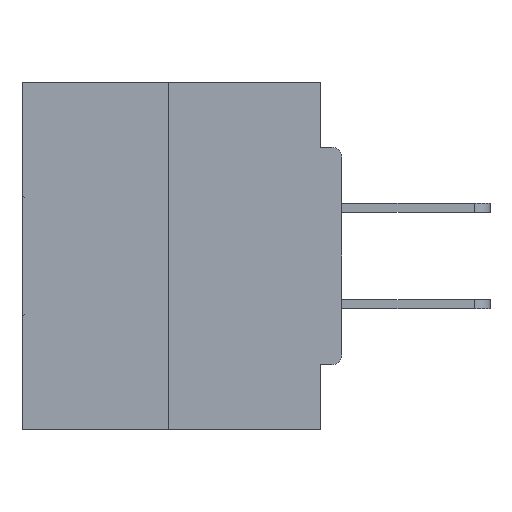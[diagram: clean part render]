
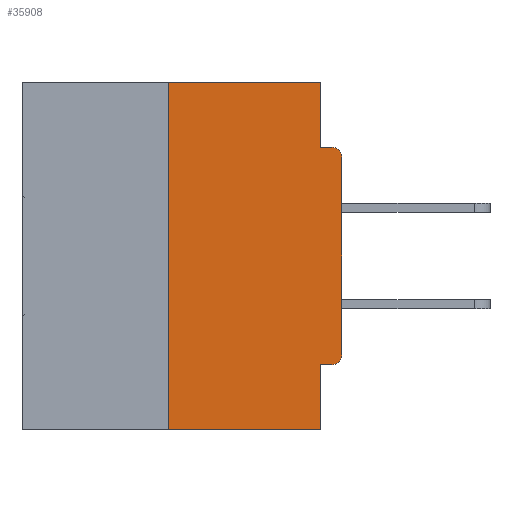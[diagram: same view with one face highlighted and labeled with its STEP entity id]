
A CAD part, left-side view. The second image highlights one B-rep face of the part: STEP entity #35908.
In plain terms, the highlighted planar face has unit normal (-1, 0, 0).
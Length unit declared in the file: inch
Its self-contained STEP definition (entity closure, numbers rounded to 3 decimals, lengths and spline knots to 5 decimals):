
#735 = DIRECTION ( 'NONE',  ( 0., 0., -1. ) ) ;
#1115 = CARTESIAN_POINT ( 'NONE',  ( 0., 0.015, -0.1085 ) ) ;
#1526 = VERTEX_POINT ( 'NONE', #32377 ) ;
#1651 = VERTEX_POINT ( 'NONE', #7397 ) ;
#2442 = VERTEX_POINT ( 'NONE', #13438 ) ;
#2557 = CARTESIAN_POINT ( 'NONE',  ( 0., 0.015, -0.3915 ) ) ;
#2795 = VECTOR ( 'NONE', #7898, 39.37008 ) ;
#3751 = CARTESIAN_POINT ( 'NONE',  ( 0., 0.46, 0. ) ) ;
#4297 = DIRECTION ( 'NONE',  ( 0., 0., -1. ) ) ;
#4385 = DIRECTION ( 'NONE',  ( 0., -1., 0. ) ) ;
#5345 = VERTEX_POINT ( 'NONE', #14491 ) ;
#5453 = ORIENTED_EDGE ( 'NONE', *, *, #39356, .F. ) ;
#5475 = VECTOR ( 'NONE', #6948, 39.37008 ) ;
#5560 = ORIENTED_EDGE ( 'NONE', *, *, #26985, .F. ) ;
#6014 = EDGE_CURVE ( 'NONE', #1651, #27121, #31995, .T. ) ;
#6642 = VERTEX_POINT ( 'NONE', #15636 ) ;
#6948 = DIRECTION ( 'NONE',  ( 0., -1., 0. ) ) ;
#7265 = CARTESIAN_POINT ( 'NONE',  ( 0., 0., -0.0935 ) ) ;
#7397 = CARTESIAN_POINT ( 'NONE',  ( 0., 0.031, -0.4065 ) ) ;
#7898 = DIRECTION ( 'NONE',  ( 0., 0., 1. ) ) ;
#8915 = DIRECTION ( 'NONE',  ( 0., 0., -1. ) ) ;
#11739 = VECTOR ( 'NONE', #20218, 39.37008 ) ;
#12076 = ORIENTED_EDGE ( 'NONE', *, *, #40522, .F. ) ;
#12921 = VERTEX_POINT ( 'NONE', #23394 ) ;
#13438 = CARTESIAN_POINT ( 'NONE',  ( 0., 0., -0.1085 ) ) ;
#13811 = LINE ( 'NONE', #32747, #17772 ) ;
#13904 = LINE ( 'NONE', #3751, #5475 ) ;
#14212 = EDGE_CURVE ( 'NONE', #17260, #2442, #13811, .T. ) ;
#14428 = DIRECTION ( 'NONE',  ( 0., 0., -1. ) ) ;
#14491 = CARTESIAN_POINT ( 'NONE',  ( 0., 0.25, 0. ) ) ;
#14674 = CIRCLE ( 'NONE', #37700, 0.015 ) ;
#14731 = VECTOR ( 'NONE', #20285, 39.37008 ) ;
#15143 = ORIENTED_EDGE ( 'NONE', *, *, #33646, .F. ) ;
#15636 = CARTESIAN_POINT ( 'NONE',  ( 0., 0.031, 0. ) ) ;
#15850 = EDGE_CURVE ( 'NONE', #18461, #17260, #14674, .T. ) ;
#16251 = DIRECTION ( 'NONE',  ( 0., 1., 0. ) ) ;
#16648 = VERTEX_POINT ( 'NONE', #29166 ) ;
#16735 = DIRECTION ( 'NONE',  ( -1., 0., 0. ) ) ;
#16987 = AXIS2_PLACEMENT_3D ( 'NONE', #17056, #20374, #14428 ) ;
#17056 = CARTESIAN_POINT ( 'NONE',  ( 0., 0.46, 0. ) ) ;
#17105 = CARTESIAN_POINT ( 'NONE',  ( 0., 0.031, -0.5 ) ) ;
#17215 = CARTESIAN_POINT ( 'NONE',  ( 0., 0.46, -0.5 ) ) ;
#17260 = VERTEX_POINT ( 'NONE', #30803 ) ;
#17595 = PLANE ( 'NONE',  #16987 ) ;
#17772 = VECTOR ( 'NONE', #39644, 39.37008 ) ;
#18461 = VERTEX_POINT ( 'NONE', #18549 ) ;
#18549 = CARTESIAN_POINT ( 'NONE',  ( 0., 0.015, -0.4065 ) ) ;
#19974 = EDGE_CURVE ( 'NONE', #2442, #12921, #27154, .T. ) ;
#20218 = DIRECTION ( 'NONE',  ( 0., -1., 0. ) ) ;
#20271 = ORIENTED_EDGE ( 'NONE', *, *, #30280, .F. ) ;
#20285 = DIRECTION ( 'NONE',  ( 0., 0., -1. ) ) ;
#20374 = DIRECTION ( 'NONE',  ( 1., 0., 0. ) ) ;
#23020 = CARTESIAN_POINT ( 'NONE',  ( 0., 0., -0.4065 ) ) ;
#23394 = CARTESIAN_POINT ( 'NONE',  ( 0., 0.015, -0.0935 ) ) ;
#24161 = CARTESIAN_POINT ( 'NONE',  ( 0., 0.25, 0. ) ) ;
#24643 = DIRECTION ( 'NONE',  ( -1., 0., 0. ) ) ;
#25325 = LINE ( 'NONE', #23020, #32210 ) ;
#25746 = ORIENTED_EDGE ( 'NONE', *, *, #19974, .T. ) ;
#26347 = LINE ( 'NONE', #35406, #37206 ) ;
#26985 = EDGE_CURVE ( 'NONE', #16648, #5345, #33568, .T. ) ;
#27121 = VERTEX_POINT ( 'NONE', #27878 ) ;
#27154 = CIRCLE ( 'NONE', #37267, 0.015 ) ;
#27878 = CARTESIAN_POINT ( 'NONE',  ( 0., 0.031, -0.5 ) ) ;
#28078 = FACE_OUTER_BOUND ( 'NONE', #37693, .T. ) ;
#28485 = EDGE_CURVE ( 'NONE', #16648, #27121, #38041, .T. ) ;
#28702 = ORIENTED_EDGE ( 'NONE', *, *, #14212, .T. ) ;
#29166 = CARTESIAN_POINT ( 'NONE',  ( 0., 0.25, -0.5 ) ) ;
#30280 = EDGE_CURVE ( 'NONE', #1526, #12921, #36443, .T. ) ;
#30803 = CARTESIAN_POINT ( 'NONE',  ( 0., 0., -0.3915 ) ) ;
#31180 = ORIENTED_EDGE ( 'NONE', *, *, #28485, .T. ) ;
#31826 = ORIENTED_EDGE ( 'NONE', *, *, #6014, .F. ) ;
#31995 = LINE ( 'NONE', #17105, #14731 ) ;
#32210 = VECTOR ( 'NONE', #16251, 39.37008 ) ;
#32377 = CARTESIAN_POINT ( 'NONE',  ( 0., 0.031, -0.0935 ) ) ;
#32747 = CARTESIAN_POINT ( 'NONE',  ( 0., 0., 0. ) ) ;
#32775 = ORIENTED_EDGE ( 'NONE', *, *, #15850, .T. ) ;
#33568 = LINE ( 'NONE', #24161, #2795 ) ;
#33646 = EDGE_CURVE ( 'NONE', #6642, #1526, #26347, .T. ) ;
#35055 = VECTOR ( 'NONE', #4385, 39.37008 ) ;
#35406 = CARTESIAN_POINT ( 'NONE',  ( 0., 0.031, 0. ) ) ;
#35908 = ADVANCED_FACE ( 'NONE', ( #28078 ), #17595, .F. ) ;
#36443 = LINE ( 'NONE', #7265, #11739 ) ;
#37206 = VECTOR ( 'NONE', #735, 39.37008 ) ;
#37267 = AXIS2_PLACEMENT_3D ( 'NONE', #1115, #16735, #4297 ) ;
#37693 = EDGE_LOOP ( 'NONE', ( #12076, #5560, #31180, #31826, #5453, #32775, #28702, #25746, #20271, #15143 ) ) ;
#37700 = AXIS2_PLACEMENT_3D ( 'NONE', #2557, #24643, #8915 ) ;
#38041 = LINE ( 'NONE', #17215, #35055 ) ;
#39356 = EDGE_CURVE ( 'NONE', #18461, #1651, #25325, .T. ) ;
#39644 = DIRECTION ( 'NONE',  ( 0., 0., 1. ) ) ;
#40522 = EDGE_CURVE ( 'NONE', #5345, #6642, #13904, .T. ) ;
